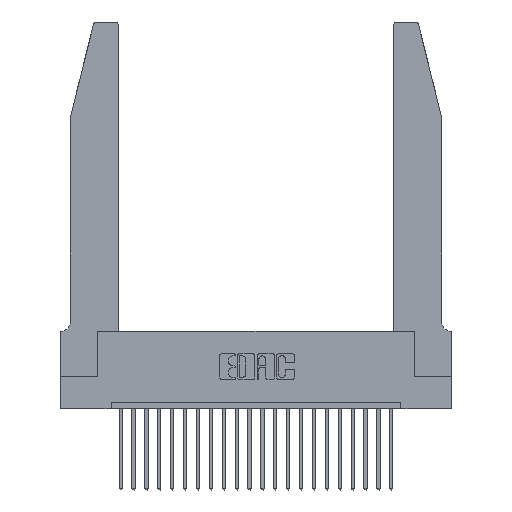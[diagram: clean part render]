
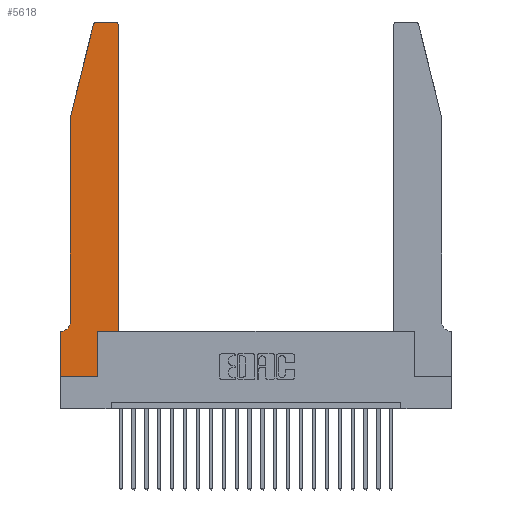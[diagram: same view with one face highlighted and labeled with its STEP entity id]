
A CAD part, top view. The second image highlights one B-rep face of the part: STEP entity #5618.
In plain terms, the highlighted planar face has unit normal (0, 0, 1).
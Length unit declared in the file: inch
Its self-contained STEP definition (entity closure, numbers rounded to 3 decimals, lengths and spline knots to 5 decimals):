
#37 = EDGE_CURVE ( 'NONE', #18109, #4698, #9131, .T. ) ;
#153 = DIRECTION ( 'NONE',  ( 0., 1., 0. ) ) ;
#391 = LINE ( 'NONE', #22182, #8788 ) ;
#443 = ORIENTED_EDGE ( 'NONE', *, *, #8080, .T. ) ;
#568 = CARTESIAN_POINT ( 'NONE',  ( 0.284, 2.72, 0.37 ) ) ;
#602 = CARTESIAN_POINT ( 'NONE',  ( 0., 0.35, 0.37 ) ) ;
#915 = VECTOR ( 'NONE', #3310, 39.37008 ) ;
#933 = LINE ( 'NONE', #14072, #18301 ) ;
#1103 = AXIS2_PLACEMENT_3D ( 'NONE', #5575, #23880, #22002 ) ;
#1186 = CARTESIAN_POINT ( 'NONE',  ( 0.2605, 2.75, 0.37 ) ) ;
#1313 = ORIENTED_EDGE ( 'NONE', *, *, #19180, .T. ) ;
#1334 = ORIENTED_EDGE ( 'NONE', *, *, #11961, .T. ) ;
#1379 = DIRECTION ( 'NONE',  ( 0., -1., 0. ) ) ;
#1411 = VERTEX_POINT ( 'NONE', #10287 ) ;
#1578 = VECTOR ( 'NONE', #12179, 39.37008 ) ;
#1620 = VERTEX_POINT ( 'NONE', #15068 ) ;
#1891 = EDGE_CURVE ( 'NONE', #3754, #17598, #933, .T. ) ;
#2248 = PLANE ( 'NONE',  #6811 ) ;
#2481 = DIRECTION ( 'NONE',  ( 0., 0., 1. ) ) ;
#2976 = CARTESIAN_POINT ( 'NONE',  ( 0.0055, 0.35, 0.37 ) ) ;
#3094 = AXIS2_PLACEMENT_3D ( 'NONE', #11867, #4287, #5977 ) ;
#3310 = DIRECTION ( 'NONE',  ( -1., 0., 0. ) ) ;
#3474 = CARTESIAN_POINT ( 'NONE',  ( 0.2865, 0.35, 0.37 ) ) ;
#3754 = VERTEX_POINT ( 'NONE', #23443 ) ;
#4287 = DIRECTION ( 'NONE',  ( 0., 0., 1. ) ) ;
#4682 = ORIENTED_EDGE ( 'NONE', *, *, #1891, .T. ) ;
#4698 = VERTEX_POINT ( 'NONE', #20472 ) ;
#4829 = FACE_OUTER_BOUND ( 'NONE', #13057, .T. ) ;
#5457 = VERTEX_POINT ( 'NONE', #13064 ) ;
#5575 = CARTESIAN_POINT ( 'NONE',  ( 0.0055, 0.42, 0.37 ) ) ;
#5618 = ADVANCED_FACE ( 'NONE', ( #4829 ), #2248, .T. ) ;
#5787 = CARTESIAN_POINT ( 'NONE',  ( 0.2865, 0., 0.37 ) ) ;
#5970 = CARTESIAN_POINT ( 'NONE',  ( 0.0755, 2., 0.37 ) ) ;
#5977 = DIRECTION ( 'NONE',  ( 1., 0., 0. ) ) ;
#6202 = DIRECTION ( 'NONE',  ( 1., 0., 0. ) ) ;
#6374 = LINE ( 'NONE', #13330, #13609 ) ;
#6778 = CIRCLE ( 'NONE', #3094, 0.03 ) ;
#6811 = AXIS2_PLACEMENT_3D ( 'NONE', #602, #2481, #6202 ) ;
#6871 = EDGE_CURVE ( 'NONE', #18659, #1620, #391, .T. ) ;
#7943 = EDGE_CURVE ( 'NONE', #8394, #1411, #11056, .T. ) ;
#8080 = EDGE_CURVE ( 'NONE', #4698, #8394, #22944, .T. ) ;
#8394 = VERTEX_POINT ( 'NONE', #2976 ) ;
#8437 = VECTOR ( 'NONE', #14638, 39.37008 ) ;
#8776 = DIRECTION ( 'NONE',  ( -1., 0., 0. ) ) ;
#8788 = VECTOR ( 'NONE', #153, 39.37008 ) ;
#9131 = LINE ( 'NONE', #5970, #15803 ) ;
#9467 = ORIENTED_EDGE ( 'NONE', *, *, #18677, .T. ) ;
#9474 = VERTEX_POINT ( 'NONE', #10007 ) ;
#9973 = DIRECTION ( 'NONE',  ( 0., 0., 1. ) ) ;
#10007 = CARTESIAN_POINT ( 'NONE',  ( 0.2865, 0.35, 0.37 ) ) ;
#10287 = CARTESIAN_POINT ( 'NONE',  ( 0., 0.35, 0.37 ) ) ;
#10324 = CARTESIAN_POINT ( 'NONE',  ( 0.4505, 0.35, 0.37 ) ) ;
#11056 = LINE ( 'NONE', #21915, #915 ) ;
#11108 = EDGE_CURVE ( 'NONE', #1411, #3754, #14351, .T. ) ;
#11187 = CARTESIAN_POINT ( 'NONE',  ( 0.284, 2.75, 0.37 ) ) ;
#11867 = CARTESIAN_POINT ( 'NONE',  ( 0.4205, 2.72, 0.37 ) ) ;
#11961 = EDGE_CURVE ( 'NONE', #1620, #20536, #6778, .T. ) ;
#12179 = DIRECTION ( 'NONE',  ( 1., 0., 0. ) ) ;
#12723 = EDGE_CURVE ( 'NONE', #13385, #5457, #14604, .T. ) ;
#13057 = EDGE_LOOP ( 'NONE', ( #23156, #16492, #1313, #22439, #443, #17247, #14405, #4682, #9467, #15675, #20238, #1334 ) ) ;
#13064 = CARTESIAN_POINT ( 'NONE',  ( 0.25487, 2.72718, 0.37 ) ) ;
#13154 = DIRECTION ( 'NONE',  ( 0., -1., 0. ) ) ;
#13330 = CARTESIAN_POINT ( 'NONE',  ( 0.0755, 2., 0.37 ) ) ;
#13385 = VERTEX_POINT ( 'NONE', #11187 ) ;
#13401 = DIRECTION ( 'NONE',  ( -0.239, -0.971, 0. ) ) ;
#13609 = VECTOR ( 'NONE', #13401, 39.37008 ) ;
#14072 = CARTESIAN_POINT ( 'NONE',  ( 0., 0., 0.37 ) ) ;
#14351 = LINE ( 'NONE', #20990, #16945 ) ;
#14405 = ORIENTED_EDGE ( 'NONE', *, *, #11108, .T. ) ;
#14604 = CIRCLE ( 'NONE', #20226, 0.03 ) ;
#14638 = DIRECTION ( 'NONE',  ( 0., 1., 0. ) ) ;
#15068 = CARTESIAN_POINT ( 'NONE',  ( 0.4505, 2.72, 0.37 ) ) ;
#15675 = ORIENTED_EDGE ( 'NONE', *, *, #17310, .T. ) ;
#15721 = DIRECTION ( 'NONE',  ( 1., 0., 0. ) ) ;
#15803 = VECTOR ( 'NONE', #13154, 39.37008 ) ;
#16492 = ORIENTED_EDGE ( 'NONE', *, *, #12723, .T. ) ;
#16659 = CARTESIAN_POINT ( 'NONE',  ( 0.4505, 0.35, 0.37 ) ) ;
#16852 = LINE ( 'NONE', #3474, #8437 ) ;
#16945 = VECTOR ( 'NONE', #1379, 39.37008 ) ;
#17247 = ORIENTED_EDGE ( 'NONE', *, *, #7943, .T. ) ;
#17310 = EDGE_CURVE ( 'NONE', #9474, #18659, #21258, .T. ) ;
#17418 = VECTOR ( 'NONE', #8776, 39.37008 ) ;
#17598 = VERTEX_POINT ( 'NONE', #5787 ) ;
#18109 = VERTEX_POINT ( 'NONE', #18795 ) ;
#18301 = VECTOR ( 'NONE', #21509, 39.37008 ) ;
#18659 = VERTEX_POINT ( 'NONE', #16659 ) ;
#18677 = EDGE_CURVE ( 'NONE', #17598, #9474, #16852, .T. ) ;
#18795 = CARTESIAN_POINT ( 'NONE',  ( 0.0755, 2., 0.37 ) ) ;
#19180 = EDGE_CURVE ( 'NONE', #5457, #18109, #6374, .T. ) ;
#20226 = AXIS2_PLACEMENT_3D ( 'NONE', #568, #9973, #15721 ) ;
#20238 = ORIENTED_EDGE ( 'NONE', *, *, #6871, .T. ) ;
#20472 = CARTESIAN_POINT ( 'NONE',  ( 0.0755, 0.42, 0.37 ) ) ;
#20536 = VERTEX_POINT ( 'NONE', #23512 ) ;
#20912 = LINE ( 'NONE', #1186, #17418 ) ;
#20990 = CARTESIAN_POINT ( 'NONE',  ( 0., 0., 0.37 ) ) ;
#21258 = LINE ( 'NONE', #10324, #1578 ) ;
#21509 = DIRECTION ( 'NONE',  ( 1., 0., 0. ) ) ;
#21915 = CARTESIAN_POINT ( 'NONE',  ( 0.0755, 0.35, 0.37 ) ) ;
#22002 = DIRECTION ( 'NONE',  ( -1., 0., 0. ) ) ;
#22182 = CARTESIAN_POINT ( 'NONE',  ( 0.4505, 0.35, 0.37 ) ) ;
#22439 = ORIENTED_EDGE ( 'NONE', *, *, #37, .T. ) ;
#22944 = CIRCLE ( 'NONE', #1103, 0.07 ) ;
#23117 = EDGE_CURVE ( 'NONE', #20536, #13385, #20912, .T. ) ;
#23156 = ORIENTED_EDGE ( 'NONE', *, *, #23117, .T. ) ;
#23443 = CARTESIAN_POINT ( 'NONE',  ( 0., 0., 0.37 ) ) ;
#23512 = CARTESIAN_POINT ( 'NONE',  ( 0.4205, 2.75, 0.37 ) ) ;
#23880 = DIRECTION ( 'NONE',  ( 0., 0., -1. ) ) ;
